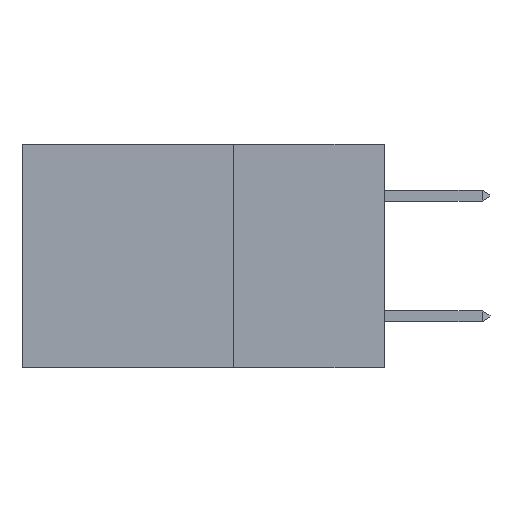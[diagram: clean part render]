
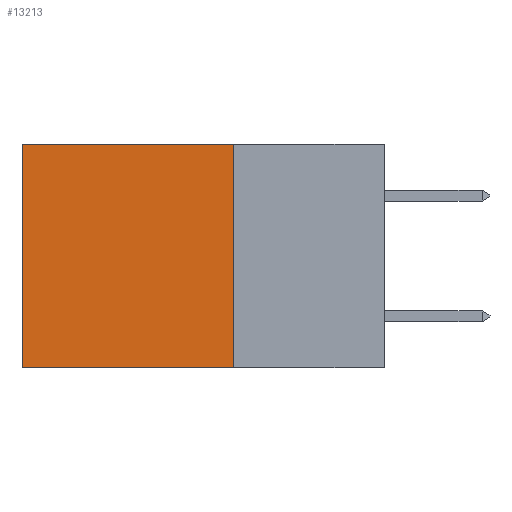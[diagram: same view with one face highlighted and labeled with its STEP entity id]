
A CAD part, left-side view. The second image highlights one B-rep face of the part: STEP entity #13213.
In plain terms, the highlighted planar face has unit normal (-1, 0, 0).
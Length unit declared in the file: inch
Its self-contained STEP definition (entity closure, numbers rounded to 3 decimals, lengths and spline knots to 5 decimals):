
#321 = CARTESIAN_POINT ( 'NONE',  ( 0.2875, 0.25, -0.37 ) ) ;
#2457 = DIRECTION ( 'NONE',  ( 0., 0., -1. ) ) ;
#2640 = CARTESIAN_POINT ( 'NONE',  ( 0.2875, 0.6, -0.37 ) ) ;
#3372 = LINE ( 'NONE', #4612, #16648 ) ;
#4160 = LINE ( 'NONE', #12120, #17795 ) ;
#4324 = CARTESIAN_POINT ( 'NONE',  ( 0.2875, 0.25, 0. ) ) ;
#4590 = ORIENTED_EDGE ( 'NONE', *, *, #16235, .F. ) ;
#4612 = CARTESIAN_POINT ( 'NONE',  ( 0.2875, 0.6, 0. ) ) ;
#5415 = PLANE ( 'NONE',  #9962 ) ;
#5836 = CARTESIAN_POINT ( 'NONE',  ( 0.2875, 0.6, 0. ) ) ;
#6683 = FACE_OUTER_BOUND ( 'NONE', #8447, .T. ) ;
#6775 = CARTESIAN_POINT ( 'NONE',  ( 0.2875, 0.25, 0. ) ) ;
#7588 = VERTEX_POINT ( 'NONE', #321 ) ;
#7728 = ORIENTED_EDGE ( 'NONE', *, *, #13714, .T. ) ;
#8102 = VERTEX_POINT ( 'NONE', #11702 ) ;
#8395 = EDGE_CURVE ( 'NONE', #7588, #16326, #14040, .T. ) ;
#8447 = EDGE_LOOP ( 'NONE', ( #7728, #11093, #4590, #10097 ) ) ;
#8915 = EDGE_CURVE ( 'NONE', #8102, #9821, #11300, .T. ) ;
#9821 = VERTEX_POINT ( 'NONE', #5836 ) ;
#9962 = AXIS2_PLACEMENT_3D ( 'NONE', #6775, #16041, #14664 ) ;
#10097 = ORIENTED_EDGE ( 'NONE', *, *, #8915, .T. ) ;
#11093 = ORIENTED_EDGE ( 'NONE', *, *, #8395, .F. ) ;
#11300 = LINE ( 'NONE', #4324, #13077 ) ;
#11415 = CARTESIAN_POINT ( 'NONE',  ( 0.2875, 0.25, -0.37 ) ) ;
#11702 = CARTESIAN_POINT ( 'NONE',  ( 0.2875, 0.25, 0. ) ) ;
#12120 = CARTESIAN_POINT ( 'NONE',  ( 0.2875, 0.25, 0. ) ) ;
#13077 = VECTOR ( 'NONE', #16849, 39.37008 ) ;
#13213 = ADVANCED_FACE ( 'NONE', ( #6683 ), #5415, .F. ) ;
#13714 = EDGE_CURVE ( 'NONE', #9821, #16326, #3372, .T. ) ;
#13936 = DIRECTION ( 'NONE',  ( 0., 1., 0. ) ) ;
#14040 = LINE ( 'NONE', #11415, #17712 ) ;
#14575 = DIRECTION ( 'NONE',  ( 0., 0., -1. ) ) ;
#14664 = DIRECTION ( 'NONE',  ( 0., 0., -1. ) ) ;
#16041 = DIRECTION ( 'NONE',  ( 1., 0., 0. ) ) ;
#16235 = EDGE_CURVE ( 'NONE', #8102, #7588, #4160, .T. ) ;
#16326 = VERTEX_POINT ( 'NONE', #2640 ) ;
#16648 = VECTOR ( 'NONE', #14575, 39.37008 ) ;
#16849 = DIRECTION ( 'NONE',  ( 0., 1., 0. ) ) ;
#17712 = VECTOR ( 'NONE', #13936, 39.37008 ) ;
#17795 = VECTOR ( 'NONE', #2457, 39.37008 ) ;
